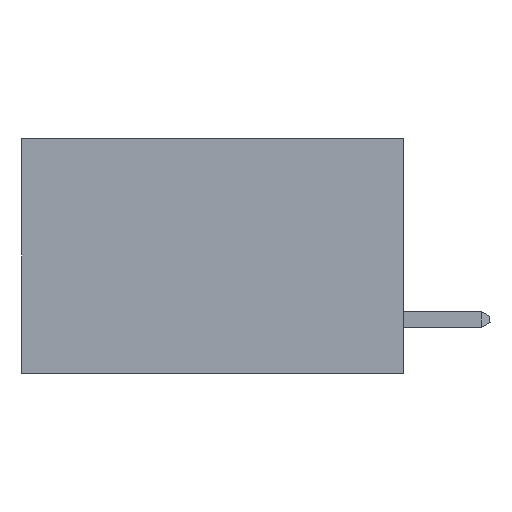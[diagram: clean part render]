
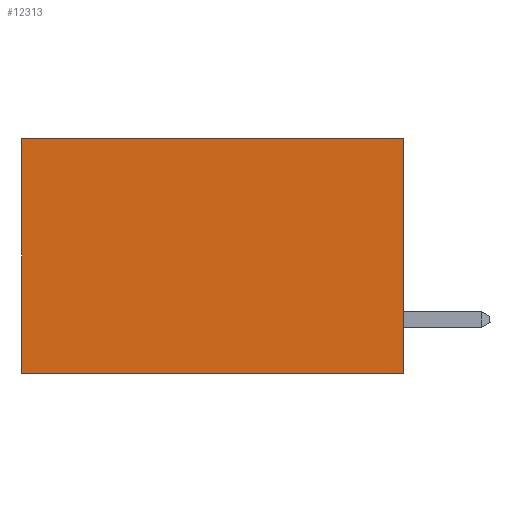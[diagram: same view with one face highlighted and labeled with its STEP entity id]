
A CAD part, left-side view. The second image highlights one B-rep face of the part: STEP entity #12313.
In plain terms, the highlighted planar face has unit normal (-1, 0, 0).
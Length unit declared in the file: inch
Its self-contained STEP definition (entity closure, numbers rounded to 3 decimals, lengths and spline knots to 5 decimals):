
#154 = LINE ( 'NONE', #3406, #1488 ) ;
#380 = ORIENTED_EDGE ( 'NONE', *, *, #1442, .F. ) ;
#525 = ORIENTED_EDGE ( 'NONE', *, *, #567, .T. ) ;
#567 = EDGE_CURVE ( 'NONE', #6371, #11031, #154, .T. ) ;
#690 = LINE ( 'NONE', #4040, #7408 ) ;
#1259 = LINE ( 'NONE', #12964, #9701 ) ;
#1442 = EDGE_CURVE ( 'NONE', #9214, #13194, #9341, .T. ) ;
#1459 = EDGE_CURVE ( 'NONE', #13194, #11031, #690, .T. ) ;
#1488 = VECTOR ( 'NONE', #14509, 39.37008 ) ;
#2424 = CARTESIAN_POINT ( 'NONE',  ( 0.2875, 0., 0. ) ) ;
#3406 = CARTESIAN_POINT ( 'NONE',  ( 0.2875, 0.6, 0. ) ) ;
#3534 = DIRECTION ( 'NONE',  ( 0., 0., -1. ) ) ;
#3746 = CARTESIAN_POINT ( 'NONE',  ( 0.2875, 0., 0. ) ) ;
#3798 = PLANE ( 'NONE',  #7562 ) ;
#4040 = CARTESIAN_POINT ( 'NONE',  ( 0.2875, 0., -0.37 ) ) ;
#4564 = EDGE_CURVE ( 'NONE', #9214, #6371, #1259, .T. ) ;
#4668 = CARTESIAN_POINT ( 'NONE',  ( 0.2875, 0.6, 0. ) ) ;
#5862 = DIRECTION ( 'NONE',  ( 0., 1., 0. ) ) ;
#5919 = CARTESIAN_POINT ( 'NONE',  ( 0.2875, 0., -0.37 ) ) ;
#6371 = VERTEX_POINT ( 'NONE', #4668 ) ;
#7408 = VECTOR ( 'NONE', #5862, 39.37008 ) ;
#7562 = AXIS2_PLACEMENT_3D ( 'NONE', #3746, #14855, #13568 ) ;
#7768 = CARTESIAN_POINT ( 'NONE',  ( 0.2875, 0., 0. ) ) ;
#9214 = VERTEX_POINT ( 'NONE', #7768 ) ;
#9341 = LINE ( 'NONE', #2424, #10510 ) ;
#9701 = VECTOR ( 'NONE', #15307, 39.37008 ) ;
#10510 = VECTOR ( 'NONE', #3534, 39.37008 ) ;
#11031 = VERTEX_POINT ( 'NONE', #11769 ) ;
#11769 = CARTESIAN_POINT ( 'NONE',  ( 0.2875, 0.6, -0.37 ) ) ;
#12153 = EDGE_LOOP ( 'NONE', ( #525, #13438, #380, #12627 ) ) ;
#12313 = ADVANCED_FACE ( 'NONE', ( #14282 ), #3798, .F. ) ;
#12627 = ORIENTED_EDGE ( 'NONE', *, *, #4564, .T. ) ;
#12964 = CARTESIAN_POINT ( 'NONE',  ( 0.2875, 0., 0. ) ) ;
#13194 = VERTEX_POINT ( 'NONE', #5919 ) ;
#13438 = ORIENTED_EDGE ( 'NONE', *, *, #1459, .F. ) ;
#13568 = DIRECTION ( 'NONE',  ( 0., 0., -1. ) ) ;
#14282 = FACE_OUTER_BOUND ( 'NONE', #12153, .T. ) ;
#14509 = DIRECTION ( 'NONE',  ( 0., 0., -1. ) ) ;
#14855 = DIRECTION ( 'NONE',  ( 1., 0., 0. ) ) ;
#15307 = DIRECTION ( 'NONE',  ( 0., 1., 0. ) ) ;
